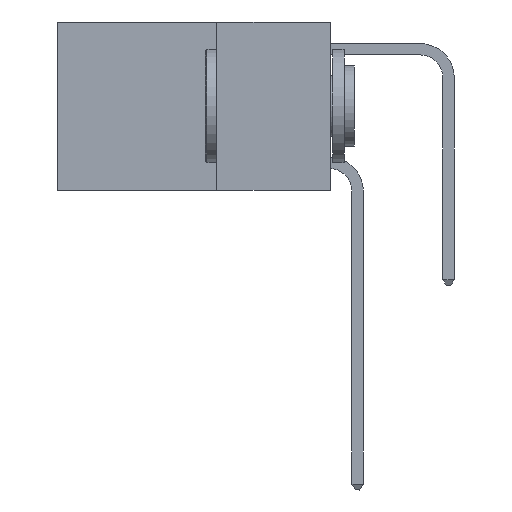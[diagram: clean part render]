
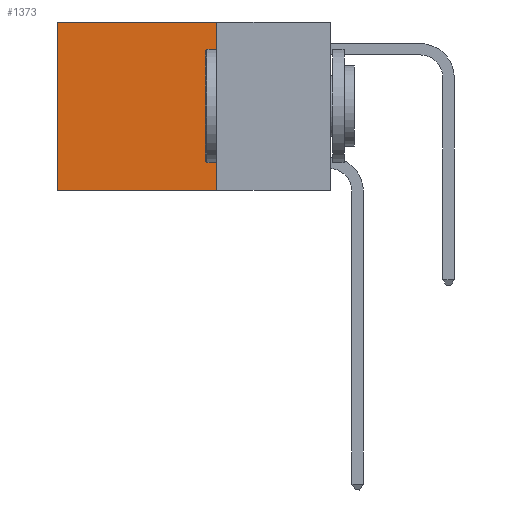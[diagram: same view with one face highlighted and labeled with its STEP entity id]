
A CAD part, left-side view. The second image highlights one B-rep face of the part: STEP entity #1373.
In plain terms, the highlighted planar face has unit normal (-1, 0, 0).
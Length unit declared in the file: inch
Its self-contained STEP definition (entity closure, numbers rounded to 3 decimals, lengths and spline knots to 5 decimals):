
#239 = VERTEX_POINT ( 'NONE', #22117 ) ;
#1373 = ADVANCED_FACE ( 'NONE', ( #12952 ), #17152, .F. ) ;
#1555 = ORIENTED_EDGE ( 'NONE', *, *, #22114, .F. ) ;
#1739 = DIRECTION ( 'NONE',  ( 0., 1., 0. ) ) ;
#1954 = ORIENTED_EDGE ( 'NONE', *, *, #12763, .T. ) ;
#2144 = AXIS2_PLACEMENT_3D ( 'NONE', #8560, #13214, #6185 ) ;
#2378 = VERTEX_POINT ( 'NONE', #13035 ) ;
#2826 = VECTOR ( 'NONE', #5790, 39.37008 ) ;
#3883 = CARTESIAN_POINT ( 'NONE',  ( 0.2625, 0.6, 0. ) ) ;
#4085 = CARTESIAN_POINT ( 'NONE',  ( 0.2625, 0.25, 0. ) ) ;
#5176 = CARTESIAN_POINT ( 'NONE',  ( 0.2625, 0.6, -0.37 ) ) ;
#5544 = LINE ( 'NONE', #24641, #14034 ) ;
#5790 = DIRECTION ( 'NONE',  ( 0., 1., 0. ) ) ;
#6185 = DIRECTION ( 'NONE',  ( 0., 0., -1. ) ) ;
#7683 = VERTEX_POINT ( 'NONE', #8292 ) ;
#7862 = VERTEX_POINT ( 'NONE', #5176 ) ;
#8292 = CARTESIAN_POINT ( 'NONE',  ( 0.2625, 0.25, 0. ) ) ;
#8560 = CARTESIAN_POINT ( 'NONE',  ( 0.2625, 0.25, 0. ) ) ;
#10837 = VECTOR ( 'NONE', #1739, 39.37008 ) ;
#11374 = ORIENTED_EDGE ( 'NONE', *, *, #12335, .T. ) ;
#12025 = DIRECTION ( 'NONE',  ( 0., 0., -1. ) ) ;
#12195 = VECTOR ( 'NONE', #17359, 39.37008 ) ;
#12335 = EDGE_CURVE ( 'NONE', #7683, #239, #23306, .T. ) ;
#12763 = EDGE_CURVE ( 'NONE', #239, #7862, #13787, .T. ) ;
#12952 = FACE_OUTER_BOUND ( 'NONE', #26261, .T. ) ;
#13035 = CARTESIAN_POINT ( 'NONE',  ( 0.2625, 0.25, -0.37 ) ) ;
#13214 = DIRECTION ( 'NONE',  ( 1., 0., 0. ) ) ;
#13787 = LINE ( 'NONE', #3883, #12195 ) ;
#14034 = VECTOR ( 'NONE', #12025, 39.37008 ) ;
#17152 = PLANE ( 'NONE',  #2144 ) ;
#17359 = DIRECTION ( 'NONE',  ( 0., 0., -1. ) ) ;
#17832 = ORIENTED_EDGE ( 'NONE', *, *, #21525, .F. ) ;
#21097 = LINE ( 'NONE', #22906, #2826 ) ;
#21525 = EDGE_CURVE ( 'NONE', #7683, #2378, #5544, .T. ) ;
#22114 = EDGE_CURVE ( 'NONE', #2378, #7862, #21097, .T. ) ;
#22117 = CARTESIAN_POINT ( 'NONE',  ( 0.2625, 0.6, 0. ) ) ;
#22906 = CARTESIAN_POINT ( 'NONE',  ( 0.2625, 0.25, -0.37 ) ) ;
#23306 = LINE ( 'NONE', #4085, #10837 ) ;
#24641 = CARTESIAN_POINT ( 'NONE',  ( 0.2625, 0.25, 0. ) ) ;
#26261 = EDGE_LOOP ( 'NONE', ( #1954, #1555, #17832, #11374 ) ) ;
